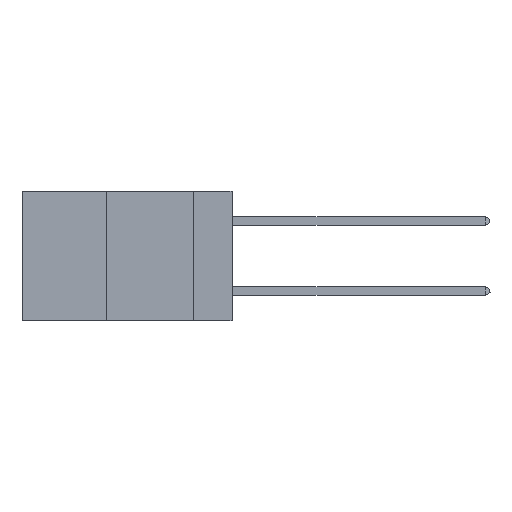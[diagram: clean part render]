
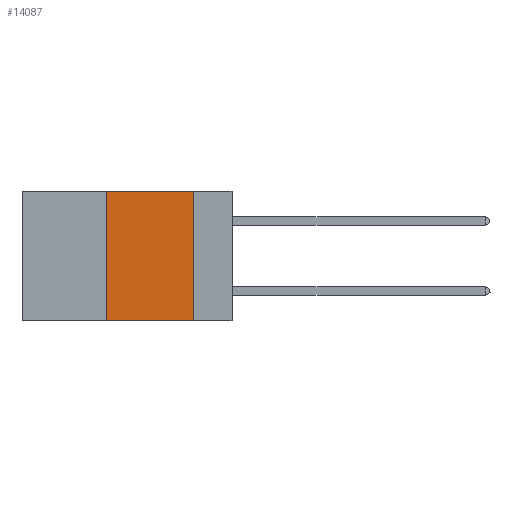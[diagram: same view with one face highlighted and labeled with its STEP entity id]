
A CAD part, left-side view. The second image highlights one B-rep face of the part: STEP entity #14087.
In plain terms, the highlighted planar face has unit normal (-1, 0, 0).
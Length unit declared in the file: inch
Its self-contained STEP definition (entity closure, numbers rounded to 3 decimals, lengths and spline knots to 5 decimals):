
#397 = CARTESIAN_POINT ( 'NONE',  ( 0., 0.36, 0. ) ) ;
#735 = VECTOR ( 'NONE', #6174, 39.37008 ) ;
#1144 = CARTESIAN_POINT ( 'NONE',  ( 0., 0.36, 0. ) ) ;
#1949 = LINE ( 'NONE', #4988, #735 ) ;
#2054 = EDGE_CURVE ( 'NONE', #13394, #13084, #1949, .T. ) ;
#2589 = CARTESIAN_POINT ( 'NONE',  ( 0., 0.11, 0. ) ) ;
#3668 = EDGE_LOOP ( 'NONE', ( #8555, #4694, #4549, #4823 ) ) ;
#3870 = CARTESIAN_POINT ( 'NONE',  ( 0., 0.11, 0. ) ) ;
#4549 = ORIENTED_EDGE ( 'NONE', *, *, #9994, .F. ) ;
#4618 = CARTESIAN_POINT ( 'NONE',  ( 0., 0.6, 0. ) ) ;
#4694 = ORIENTED_EDGE ( 'NONE', *, *, #2054, .F. ) ;
#4823 = ORIENTED_EDGE ( 'NONE', *, *, #7613, .T. ) ;
#4978 = LINE ( 'NONE', #397, #5336 ) ;
#4988 = CARTESIAN_POINT ( 'NONE',  ( 0., 0.6, 0. ) ) ;
#5336 = VECTOR ( 'NONE', #11422, 39.37008 ) ;
#5581 = CARTESIAN_POINT ( 'NONE',  ( 0., 0.6, -0.37 ) ) ;
#5833 = CARTESIAN_POINT ( 'NONE',  ( 0., 0.36, -0.37 ) ) ;
#6174 = DIRECTION ( 'NONE',  ( 0., -1., 0. ) ) ;
#6776 = VERTEX_POINT ( 'NONE', #5833 ) ;
#6858 = DIRECTION ( 'NONE',  ( 1., 0., 0. ) ) ;
#7613 = EDGE_CURVE ( 'NONE', #6776, #13285, #7674, .T. ) ;
#7674 = LINE ( 'NONE', #5581, #13839 ) ;
#8555 = ORIENTED_EDGE ( 'NONE', *, *, #11634, .F. ) ;
#8776 = DIRECTION ( 'NONE',  ( 0., -1., 0. ) ) ;
#9994 = EDGE_CURVE ( 'NONE', #6776, #13394, #4978, .T. ) ;
#10395 = AXIS2_PLACEMENT_3D ( 'NONE', #4618, #6858, #12490 ) ;
#10705 = VECTOR ( 'NONE', #11694, 39.37008 ) ;
#10888 = CARTESIAN_POINT ( 'NONE',  ( 0., 0.11, -0.37 ) ) ;
#11367 = LINE ( 'NONE', #3870, #10705 ) ;
#11422 = DIRECTION ( 'NONE',  ( 0., 0., 1. ) ) ;
#11634 = EDGE_CURVE ( 'NONE', #13084, #13285, #11367, .T. ) ;
#11694 = DIRECTION ( 'NONE',  ( 0., 0., -1. ) ) ;
#11996 = FACE_OUTER_BOUND ( 'NONE', #3668, .T. ) ;
#12446 = PLANE ( 'NONE',  #10395 ) ;
#12490 = DIRECTION ( 'NONE',  ( 0., 0., -1. ) ) ;
#13084 = VERTEX_POINT ( 'NONE', #2589 ) ;
#13285 = VERTEX_POINT ( 'NONE', #10888 ) ;
#13394 = VERTEX_POINT ( 'NONE', #1144 ) ;
#13839 = VECTOR ( 'NONE', #8776, 39.37008 ) ;
#14087 = ADVANCED_FACE ( 'NONE', ( #11996 ), #12446, .F. ) ;
